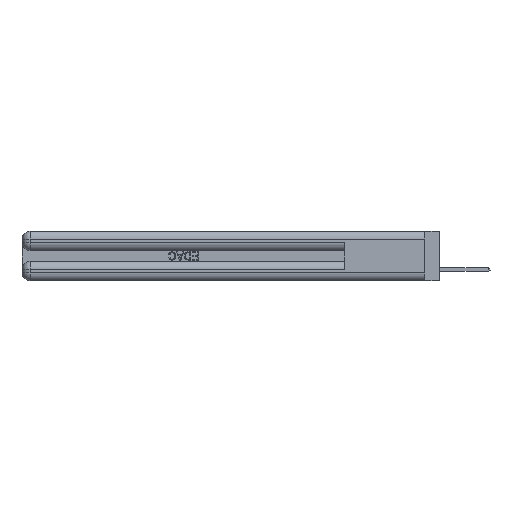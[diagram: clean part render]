
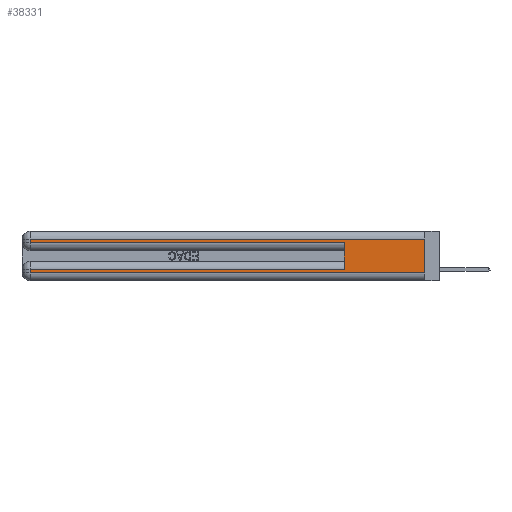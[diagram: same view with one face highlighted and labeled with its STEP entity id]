
A CAD part, left-side view. The second image highlights one B-rep face of the part: STEP entity #38331.
In plain terms, the highlighted planar face has unit normal (-1, 0, 0).
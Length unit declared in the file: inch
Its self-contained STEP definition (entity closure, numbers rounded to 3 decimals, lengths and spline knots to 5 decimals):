
#717 = DIRECTION ( 'NONE',  ( 0., 1., 0. ) ) ;
#789 = ORIENTED_EDGE ( 'NONE', *, *, #24725, .F. ) ;
#1543 = VERTEX_POINT ( 'NONE', #23843 ) ;
#1630 = EDGE_CURVE ( 'NONE', #35535, #29333, #23836, .T. ) ;
#1734 = CARTESIAN_POINT ( 'NONE',  ( 0., 0., 0.37 ) ) ;
#1990 = VECTOR ( 'NONE', #21756, 39.37008 ) ;
#2311 = LINE ( 'NONE', #19866, #12503 ) ;
#2772 = DIRECTION ( 'NONE',  ( 0., 0., -1. ) ) ;
#3238 = EDGE_CURVE ( 'NONE', #16010, #1543, #32739, .T. ) ;
#4350 = EDGE_LOOP ( 'NONE', ( #789, #24099, #18019, #6448, #34094, #41527, #8199, #37734 ) ) ;
#4925 = CARTESIAN_POINT ( 'NONE',  ( 0., 0., 0.06 ) ) ;
#5139 = CARTESIAN_POINT ( 'NONE',  ( 0., 0.6, 0.145 ) ) ;
#5204 = DIRECTION ( 'NONE',  ( 1., 0., 0. ) ) ;
#6448 = ORIENTED_EDGE ( 'NONE', *, *, #12819, .T. ) ;
#8050 = FACE_OUTER_BOUND ( 'NONE', #4350, .T. ) ;
#8199 = ORIENTED_EDGE ( 'NONE', *, *, #8299, .T. ) ;
#8299 = EDGE_CURVE ( 'NONE', #29333, #31967, #41303, .T. ) ;
#8806 = CARTESIAN_POINT ( 'NONE',  ( 0., 2.94, 0.085 ) ) ;
#8818 = VECTOR ( 'NONE', #717, 39.37008 ) ;
#9067 = CARTESIAN_POINT ( 'NONE',  ( 0., 0.6, 0.085 ) ) ;
#12503 = VECTOR ( 'NONE', #43935, 39.37008 ) ;
#12819 = EDGE_CURVE ( 'NONE', #36495, #38711, #30553, .T. ) ;
#15011 = LINE ( 'NONE', #32982, #22514 ) ;
#15625 = VECTOR ( 'NONE', #23300, 39.37008 ) ;
#16010 = VERTEX_POINT ( 'NONE', #18894 ) ;
#16447 = DIRECTION ( 'NONE',  ( 0., 1., 0. ) ) ;
#17374 = VECTOR ( 'NONE', #28941, 39.37008 ) ;
#18019 = ORIENTED_EDGE ( 'NONE', *, *, #30451, .T. ) ;
#18894 = CARTESIAN_POINT ( 'NONE',  ( 0., 0., 0.31 ) ) ;
#19778 = EDGE_CURVE ( 'NONE', #35535, #38711, #23809, .T. ) ;
#19866 = CARTESIAN_POINT ( 'NONE',  ( 0., 0., 0.06 ) ) ;
#21484 = VECTOR ( 'NONE', #16447, 39.37008 ) ;
#21756 = DIRECTION ( 'NONE',  ( 0., 0., -1. ) ) ;
#22514 = VECTOR ( 'NONE', #2772, 39.37008 ) ;
#23084 = DIRECTION ( 'NONE',  ( 0., -1., 0. ) ) ;
#23300 = DIRECTION ( 'NONE',  ( 0., 0., -1. ) ) ;
#23809 = LINE ( 'NONE', #5139, #17374 ) ;
#23836 = LINE ( 'NONE', #41446, #8818 ) ;
#23843 = CARTESIAN_POINT ( 'NONE',  ( 0., 2.94, 0.31 ) ) ;
#24099 = ORIENTED_EDGE ( 'NONE', *, *, #3238, .T. ) ;
#24725 = EDGE_CURVE ( 'NONE', #16010, #29385, #15011, .T. ) ;
#25063 = CARTESIAN_POINT ( 'NONE',  ( 0., 2.94, 0.37 ) ) ;
#26510 = CARTESIAN_POINT ( 'NONE',  ( 0., 2.94, 0.06 ) ) ;
#28941 = DIRECTION ( 'NONE',  ( 0., 0., 1. ) ) ;
#29333 = VERTEX_POINT ( 'NONE', #8806 ) ;
#29385 = VERTEX_POINT ( 'NONE', #4925 ) ;
#30421 = CARTESIAN_POINT ( 'NONE',  ( 0., 0., 0.285 ) ) ;
#30451 = EDGE_CURVE ( 'NONE', #1543, #36495, #34120, .T. ) ;
#30553 = LINE ( 'NONE', #30421, #31561 ) ;
#31561 = VECTOR ( 'NONE', #23084, 39.37008 ) ;
#31967 = VERTEX_POINT ( 'NONE', #26510 ) ;
#32739 = LINE ( 'NONE', #33648, #21484 ) ;
#32982 = CARTESIAN_POINT ( 'NONE',  ( 0., 0., 0.37 ) ) ;
#33334 = EDGE_CURVE ( 'NONE', #31967, #29385, #2311, .T. ) ;
#33648 = CARTESIAN_POINT ( 'NONE',  ( 0., 0., 0.31 ) ) ;
#34094 = ORIENTED_EDGE ( 'NONE', *, *, #19778, .F. ) ;
#34120 = LINE ( 'NONE', #25063, #1990 ) ;
#35535 = VERTEX_POINT ( 'NONE', #9067 ) ;
#36495 = VERTEX_POINT ( 'NONE', #38456 ) ;
#36947 = CARTESIAN_POINT ( 'NONE',  ( 0., 2.94, 0.37 ) ) ;
#37734 = ORIENTED_EDGE ( 'NONE', *, *, #33334, .T. ) ;
#37749 = AXIS2_PLACEMENT_3D ( 'NONE', #1734, #5204, #39465 ) ;
#38331 = ADVANCED_FACE ( 'NONE', ( #8050 ), #42757, .F. ) ;
#38456 = CARTESIAN_POINT ( 'NONE',  ( 0., 2.94, 0.285 ) ) ;
#38711 = VERTEX_POINT ( 'NONE', #41496 ) ;
#39465 = DIRECTION ( 'NONE',  ( 0., 0., -1. ) ) ;
#41303 = LINE ( 'NONE', #36947, #15625 ) ;
#41446 = CARTESIAN_POINT ( 'NONE',  ( 0., 0., 0.085 ) ) ;
#41496 = CARTESIAN_POINT ( 'NONE',  ( 0., 0.6, 0.285 ) ) ;
#41527 = ORIENTED_EDGE ( 'NONE', *, *, #1630, .T. ) ;
#42757 = PLANE ( 'NONE',  #37749 ) ;
#43935 = DIRECTION ( 'NONE',  ( 0., -1., 0. ) ) ;
